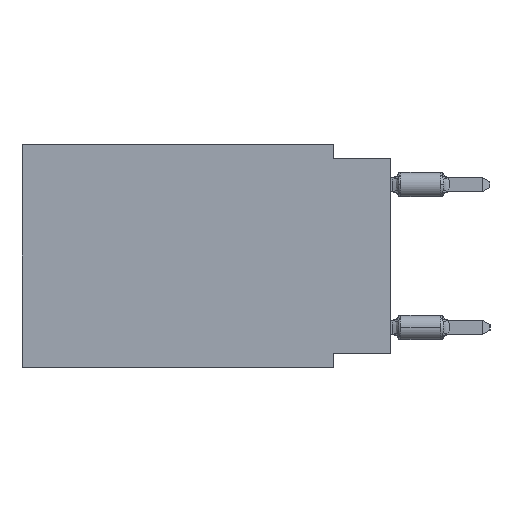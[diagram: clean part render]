
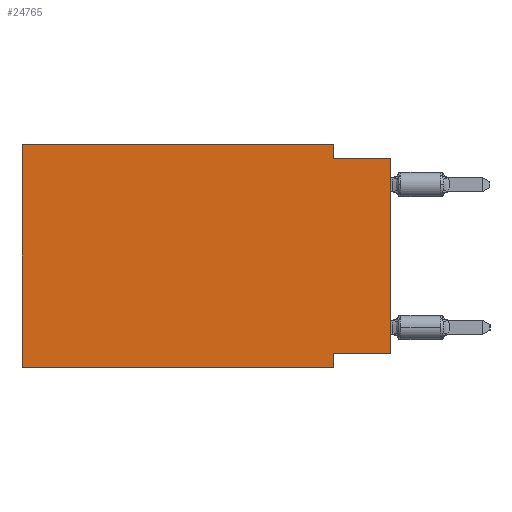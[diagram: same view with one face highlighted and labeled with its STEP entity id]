
A CAD part, left-side view. The second image highlights one B-rep face of the part: STEP entity #24765.
In plain terms, the highlighted planar face has unit normal (-1, 0, 0).
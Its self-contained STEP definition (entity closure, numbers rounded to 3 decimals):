
#479 = EDGE_CURVE ( 'NONE', #1857, #7326, #30448, .T. ) ;
#701 = LINE ( 'NONE', #28252, #34561 ) ;
#923 = DIRECTION ( 'NONE',  ( 0., 0., -1. ) ) ;
#1857 = VERTEX_POINT ( 'NONE', #20161 ) ;
#3423 = CARTESIAN_POINT ( 'NONE',  ( 0., 16.383, 0. ) ) ;
#5730 = EDGE_CURVE ( 'NONE', #7326, #27194, #30629, .T. ) ;
#5931 = CARTESIAN_POINT ( 'NONE',  ( 0., 16.383, 0. ) ) ;
#6072 = LINE ( 'NONE', #11260, #18906 ) ;
#6248 = DIRECTION ( 'NONE',  ( 0., -1., 0. ) ) ;
#6684 = ORIENTED_EDGE ( 'NONE', *, *, #13782, .T. ) ;
#7326 = VERTEX_POINT ( 'NONE', #29442 ) ;
#7906 = EDGE_CURVE ( 'NONE', #29000, #12315, #6072, .T. ) ;
#8091 = DIRECTION ( 'NONE',  ( 0., 0., 1. ) ) ;
#9751 = CARTESIAN_POINT ( 'NONE',  ( 0., 0., -9.271 ) ) ;
#10834 = VECTOR ( 'NONE', #8091, 1000. ) ;
#10842 = ORIENTED_EDGE ( 'NONE', *, *, #5730, .F. ) ;
#11214 = VECTOR ( 'NONE', #15646, 1000. ) ;
#11260 = CARTESIAN_POINT ( 'NONE',  ( 0., 0., -0.635 ) ) ;
#11913 = DIRECTION ( 'NONE',  ( 0., -1., 0. ) ) ;
#12315 = VERTEX_POINT ( 'NONE', #21869 ) ;
#12404 = DIRECTION ( 'NONE',  ( 1., 0., 0. ) ) ;
#12761 = PLANE ( 'NONE',  #32669 ) ;
#12795 = LINE ( 'NONE', #26572, #11214 ) ;
#13782 = EDGE_CURVE ( 'NONE', #17200, #12315, #701, .T. ) ;
#13791 = VECTOR ( 'NONE', #21701, 1000. ) ;
#14115 = EDGE_CURVE ( 'NONE', #1857, #23383, #20158, .T. ) ;
#14331 = LINE ( 'NONE', #22043, #14959 ) ;
#14461 = DIRECTION ( 'NONE',  ( 0., 0., 1. ) ) ;
#14915 = CARTESIAN_POINT ( 'NONE',  ( 0., 16.383, 0. ) ) ;
#14959 = VECTOR ( 'NONE', #923, 1000. ) ;
#15258 = FACE_OUTER_BOUND ( 'NONE', #17183, .T. ) ;
#15646 = DIRECTION ( 'NONE',  ( 0., 0., -1. ) ) ;
#17013 = VECTOR ( 'NONE', #22729, 1000. ) ;
#17183 = EDGE_LOOP ( 'NONE', ( #6684, #30312, #30118, #10842, #30114, #20124, #33324, #31275 ) ) ;
#17200 = VERTEX_POINT ( 'NONE', #9751 ) ;
#18509 = CARTESIAN_POINT ( 'NONE',  ( 0., 2.54, -9.271 ) ) ;
#18845 = LINE ( 'NONE', #21529, #13791 ) ;
#18906 = VECTOR ( 'NONE', #6248, 1000. ) ;
#19592 = CARTESIAN_POINT ( 'NONE',  ( 0., 2.54, -9.906 ) ) ;
#20124 = ORIENTED_EDGE ( 'NONE', *, *, #14115, .T. ) ;
#20158 = LINE ( 'NONE', #31079, #24306 ) ;
#20161 = CARTESIAN_POINT ( 'NONE',  ( 0., 16.383, -9.906 ) ) ;
#20293 = DIRECTION ( 'NONE',  ( 0., 0., -1. ) ) ;
#21529 = CARTESIAN_POINT ( 'NONE',  ( 0., 0., -9.271 ) ) ;
#21701 = DIRECTION ( 'NONE',  ( 0., 1., 0. ) ) ;
#21869 = CARTESIAN_POINT ( 'NONE',  ( 0., 0., -0.635 ) ) ;
#22043 = CARTESIAN_POINT ( 'NONE',  ( 0., 2.54, -9.906 ) ) ;
#22729 = DIRECTION ( 'NONE',  ( 0., -1., 0. ) ) ;
#23383 = VERTEX_POINT ( 'NONE', #19592 ) ;
#23707 = EDGE_CURVE ( 'NONE', #29660, #23383, #14331, .T. ) ;
#24306 = VECTOR ( 'NONE', #11913, 1000. ) ;
#24765 = ADVANCED_FACE ( 'NONE', ( #15258 ), #12761, .F. ) ;
#24911 = EDGE_CURVE ( 'NONE', #17200, #29660, #18845, .T. ) ;
#26572 = CARTESIAN_POINT ( 'NONE',  ( 0., 2.54, 0. ) ) ;
#27194 = VERTEX_POINT ( 'NONE', #28541 ) ;
#28252 = CARTESIAN_POINT ( 'NONE',  ( 0., 0., 0. ) ) ;
#28541 = CARTESIAN_POINT ( 'NONE',  ( 0., 2.54, 0. ) ) ;
#29000 = VERTEX_POINT ( 'NONE', #35124 ) ;
#29442 = CARTESIAN_POINT ( 'NONE',  ( 0., 16.383, 0. ) ) ;
#29577 = EDGE_CURVE ( 'NONE', #27194, #29000, #12795, .T. ) ;
#29660 = VERTEX_POINT ( 'NONE', #18509 ) ;
#30114 = ORIENTED_EDGE ( 'NONE', *, *, #479, .F. ) ;
#30118 = ORIENTED_EDGE ( 'NONE', *, *, #29577, .F. ) ;
#30312 = ORIENTED_EDGE ( 'NONE', *, *, #7906, .F. ) ;
#30448 = LINE ( 'NONE', #5931, #10834 ) ;
#30629 = LINE ( 'NONE', #3423, #17013 ) ;
#31079 = CARTESIAN_POINT ( 'NONE',  ( 0., 16.383, -9.906 ) ) ;
#31275 = ORIENTED_EDGE ( 'NONE', *, *, #24911, .F. ) ;
#32669 = AXIS2_PLACEMENT_3D ( 'NONE', #14915, #12404, #20293 ) ;
#33324 = ORIENTED_EDGE ( 'NONE', *, *, #23707, .F. ) ;
#34561 = VECTOR ( 'NONE', #14461, 1000. ) ;
#35124 = CARTESIAN_POINT ( 'NONE',  ( 0., 2.54, -0.635 ) ) ;
